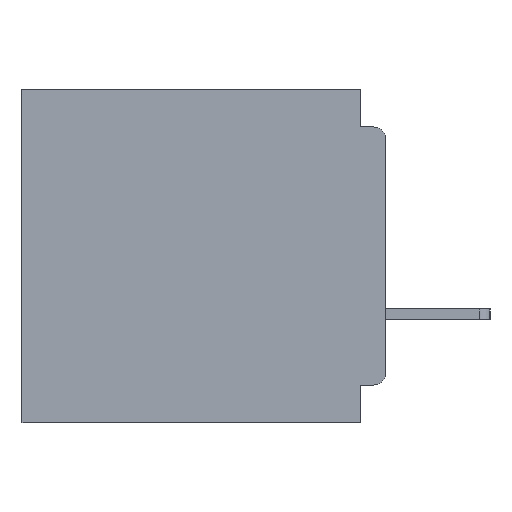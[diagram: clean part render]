
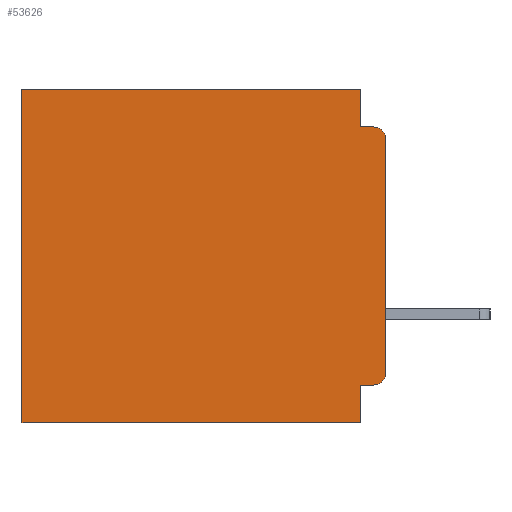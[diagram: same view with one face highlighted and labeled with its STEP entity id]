
A CAD part, left-side view. The second image highlights one B-rep face of the part: STEP entity #53626.
In plain terms, the highlighted planar face has unit normal (-1, 0, 0).
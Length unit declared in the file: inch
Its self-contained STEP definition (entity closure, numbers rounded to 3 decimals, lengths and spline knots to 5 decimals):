
#57 = PLANE ( 'NONE',  #8849 ) ;
#1054 = ORIENTED_EDGE ( 'NONE', *, *, #53941, .F. ) ;
#1423 = VERTEX_POINT ( 'NONE', #9544 ) ;
#1960 = EDGE_CURVE ( 'NONE', #17098, #9258, #18657, .T. ) ;
#3105 = ORIENTED_EDGE ( 'NONE', *, *, #53214, .T. ) ;
#3529 = CARTESIAN_POINT ( 'NONE',  ( 0.3, 0., -0.355 ) ) ;
#4558 = DIRECTION ( 'NONE',  ( 1., 0., 0. ) ) ;
#4599 = DIRECTION ( 'NONE',  ( 0., 1., 0. ) ) ;
#5092 = CARTESIAN_POINT ( 'NONE',  ( 0.3, 0.437, -0.4 ) ) ;
#5851 = CARTESIAN_POINT ( 'NONE',  ( 0.3, 0.437, -0.4 ) ) ;
#6140 = VECTOR ( 'NONE', #46013, 39.37008 ) ;
#7330 = CARTESIAN_POINT ( 'NONE',  ( 0.3, 0., -0.045 ) ) ;
#7483 = VECTOR ( 'NONE', #4599, 39.37008 ) ;
#8558 = EDGE_CURVE ( 'NONE', #9641, #28432, #41395, .T. ) ;
#8792 = VECTOR ( 'NONE', #26586, 39.37008 ) ;
#8849 = AXIS2_PLACEMENT_3D ( 'NONE', #35573, #4558, #35763 ) ;
#9258 = VERTEX_POINT ( 'NONE', #56902 ) ;
#9544 = CARTESIAN_POINT ( 'NONE',  ( 0.3, 0.031, -0.355 ) ) ;
#9641 = VERTEX_POINT ( 'NONE', #33938 ) ;
#10106 = LINE ( 'NONE', #7330, #55927 ) ;
#10374 = CARTESIAN_POINT ( 'NONE',  ( 0.3, 0.015, -0.355 ) ) ;
#10655 = DIRECTION ( 'NONE',  ( -1., 0., 0. ) ) ;
#11323 = EDGE_CURVE ( 'NONE', #9258, #24788, #28521, .T. ) ;
#11394 = ORIENTED_EDGE ( 'NONE', *, *, #26802, .F. ) ;
#12027 = DIRECTION ( 'NONE',  ( 0., -1., 0. ) ) ;
#13653 = EDGE_CURVE ( 'NONE', #17098, #47025, #21722, .T. ) ;
#14334 = CARTESIAN_POINT ( 'NONE',  ( 0.3, 0.031, -0.045 ) ) ;
#15154 = CIRCLE ( 'NONE', #49810, 0.015 ) ;
#16026 = ORIENTED_EDGE ( 'NONE', *, *, #53127, .F. ) ;
#16282 = VECTOR ( 'NONE', #40293, 39.37008 ) ;
#17098 = VERTEX_POINT ( 'NONE', #39914 ) ;
#17239 = VECTOR ( 'NONE', #37133, 39.37008 ) ;
#17279 = ORIENTED_EDGE ( 'NONE', *, *, #8558, .F. ) ;
#18657 = LINE ( 'NONE', #25734, #17239 ) ;
#19984 = CARTESIAN_POINT ( 'NONE',  ( 0.3, 0.015, -0.06 ) ) ;
#21722 = LINE ( 'NONE', #23915, #55604 ) ;
#23069 = VERTEX_POINT ( 'NONE', #41158 ) ;
#23370 = VECTOR ( 'NONE', #48102, 39.37008 ) ;
#23915 = CARTESIAN_POINT ( 'NONE',  ( 0.3, 0.031, 0. ) ) ;
#24274 = FACE_OUTER_BOUND ( 'NONE', #39642, .T. ) ;
#24482 = DIRECTION ( 'NONE',  ( 0., 0., -1. ) ) ;
#24788 = VERTEX_POINT ( 'NONE', #5092 ) ;
#25734 = CARTESIAN_POINT ( 'NONE',  ( 0.3, 0., 0. ) ) ;
#26388 = CIRCLE ( 'NONE', #50927, 0.015 ) ;
#26586 = DIRECTION ( 'NONE',  ( 0., 0., -1. ) ) ;
#26802 = EDGE_CURVE ( 'NONE', #47025, #46866, #10106, .T. ) ;
#27226 = ORIENTED_EDGE ( 'NONE', *, *, #13653, .F. ) ;
#28432 = VERTEX_POINT ( 'NONE', #50925 ) ;
#28521 = LINE ( 'NONE', #5851, #6140 ) ;
#28915 = LINE ( 'NONE', #3529, #23370 ) ;
#32769 = ORIENTED_EDGE ( 'NONE', *, *, #40706, .F. ) ;
#32903 = ORIENTED_EDGE ( 'NONE', *, *, #1960, .T. ) ;
#33570 = EDGE_CURVE ( 'NONE', #9641, #46866, #26388, .T. ) ;
#33743 = ORIENTED_EDGE ( 'NONE', *, *, #11323, .T. ) ;
#33938 = CARTESIAN_POINT ( 'NONE',  ( 0.3, 0., -0.06 ) ) ;
#35573 = CARTESIAN_POINT ( 'NONE',  ( 0.3, 0., -0.4 ) ) ;
#35763 = DIRECTION ( 'NONE',  ( 0., 0., -1. ) ) ;
#36776 = VERTEX_POINT ( 'NONE', #10374 ) ;
#37133 = DIRECTION ( 'NONE',  ( 0., 1., 0. ) ) ;
#37386 = CARTESIAN_POINT ( 'NONE',  ( 0.3, 0.015, -0.34 ) ) ;
#37659 = ORIENTED_EDGE ( 'NONE', *, *, #33570, .T. ) ;
#39642 = EDGE_LOOP ( 'NONE', ( #17279, #37659, #11394, #27226, #32903, #33743, #16026, #1054, #32769, #3105 ) ) ;
#39914 = CARTESIAN_POINT ( 'NONE',  ( 0.3, 0.031, 0. ) ) ;
#40271 = CARTESIAN_POINT ( 'NONE',  ( 0.3, 0., -0.4 ) ) ;
#40293 = DIRECTION ( 'NONE',  ( 0., 0., -1. ) ) ;
#40706 = EDGE_CURVE ( 'NONE', #36776, #1423, #28915, .T. ) ;
#41158 = CARTESIAN_POINT ( 'NONE',  ( 0.3, 0.031, -0.4 ) ) ;
#41395 = LINE ( 'NONE', #44801, #16282 ) ;
#41851 = DIRECTION ( 'NONE',  ( 0., 0., -1. ) ) ;
#44801 = CARTESIAN_POINT ( 'NONE',  ( 0.3, 0., -0.4 ) ) ;
#46013 = DIRECTION ( 'NONE',  ( 0., 0., -1. ) ) ;
#46230 = DIRECTION ( 'NONE',  ( 0., 0., -1. ) ) ;
#46866 = VERTEX_POINT ( 'NONE', #48754 ) ;
#47025 = VERTEX_POINT ( 'NONE', #14334 ) ;
#48102 = DIRECTION ( 'NONE',  ( 0., 1., 0. ) ) ;
#48754 = CARTESIAN_POINT ( 'NONE',  ( 0.3, 0.015, -0.045 ) ) ;
#49810 = AXIS2_PLACEMENT_3D ( 'NONE', #37386, #10655, #41851 ) ;
#50925 = CARTESIAN_POINT ( 'NONE',  ( 0.3, 0., -0.34 ) ) ;
#50927 = AXIS2_PLACEMENT_3D ( 'NONE', #19984, #50987, #24482 ) ;
#50987 = DIRECTION ( 'NONE',  ( -1., 0., 0. ) ) ;
#53127 = EDGE_CURVE ( 'NONE', #23069, #24788, #53377, .T. ) ;
#53214 = EDGE_CURVE ( 'NONE', #36776, #28432, #15154, .T. ) ;
#53377 = LINE ( 'NONE', #40271, #7483 ) ;
#53626 = ADVANCED_FACE ( 'NONE', ( #24274 ), #57, .F. ) ;
#53941 = EDGE_CURVE ( 'NONE', #1423, #23069, #56014, .T. ) ;
#55604 = VECTOR ( 'NONE', #46230, 39.37008 ) ;
#55927 = VECTOR ( 'NONE', #12027, 39.37008 ) ;
#56014 = LINE ( 'NONE', #57439, #8792 ) ;
#56902 = CARTESIAN_POINT ( 'NONE',  ( 0.3, 0.437, 0. ) ) ;
#57439 = CARTESIAN_POINT ( 'NONE',  ( 0.3, 0.031, -0.4 ) ) ;
